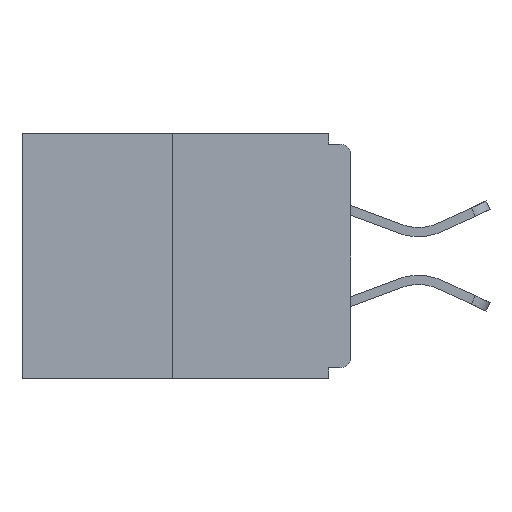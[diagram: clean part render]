
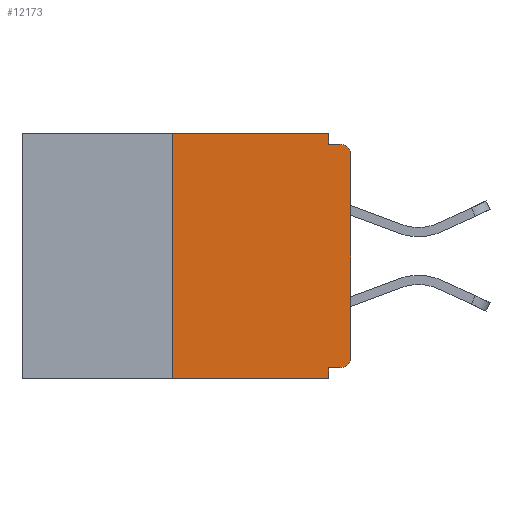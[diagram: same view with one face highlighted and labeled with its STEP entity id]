
A CAD part, left-side view. The second image highlights one B-rep face of the part: STEP entity #12173.
In plain terms, the highlighted planar face has unit normal (-1, 0, 0).
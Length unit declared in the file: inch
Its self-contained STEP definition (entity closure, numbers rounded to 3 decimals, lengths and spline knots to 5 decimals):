
#519 = VERTEX_POINT ( 'NONE', #11648 ) ;
#792 = VERTEX_POINT ( 'NONE', #8527 ) ;
#1219 = LINE ( 'NONE', #9843, #12576 ) ;
#1291 = CARTESIAN_POINT ( 'NONE',  ( 0., 0.25, 0. ) ) ;
#1317 = ORIENTED_EDGE ( 'NONE', *, *, #2907, .F. ) ;
#1701 = VERTEX_POINT ( 'NONE', #1969 ) ;
#1830 = CIRCLE ( 'NONE', #7094, 0.015 ) ;
#1933 = DIRECTION ( 'NONE',  ( -1., 0., 0. ) ) ;
#1969 = CARTESIAN_POINT ( 'NONE',  ( 0., 0.25, 0. ) ) ;
#2136 = ORIENTED_EDGE ( 'NONE', *, *, #7452, .T. ) ;
#2603 = CARTESIAN_POINT ( 'NONE',  ( 0., 0.25, -0.343 ) ) ;
#2713 = LINE ( 'NONE', #6133, #3054 ) ;
#2848 = FACE_OUTER_BOUND ( 'NONE', #6129, .T. ) ;
#2907 = EDGE_CURVE ( 'NONE', #4086, #519, #5922, .T. ) ;
#2918 = EDGE_CURVE ( 'NONE', #12275, #792, #8336, .T. ) ;
#2997 = DIRECTION ( 'NONE',  ( 0., 0., -1. ) ) ;
#3054 = VECTOR ( 'NONE', #9433, 39.37008 ) ;
#3148 = VECTOR ( 'NONE', #2997, 39.37008 ) ;
#3778 = CARTESIAN_POINT ( 'NONE',  ( 0., 0., -0.328 ) ) ;
#4086 = VERTEX_POINT ( 'NONE', #12281 ) ;
#4287 = CARTESIAN_POINT ( 'NONE',  ( 0., 0., -0.015 ) ) ;
#4357 = CARTESIAN_POINT ( 'NONE',  ( 0., 0.015, -0.03 ) ) ;
#4374 = DIRECTION ( 'NONE',  ( 0., -1., 0. ) ) ;
#4580 = CARTESIAN_POINT ( 'NONE',  ( 0., 0.015, -0.015 ) ) ;
#4688 = EDGE_CURVE ( 'NONE', #11669, #1701, #9485, .T. ) ;
#4873 = DIRECTION ( 'NONE',  ( 0., 1., 0. ) ) ;
#5019 = CARTESIAN_POINT ( 'NONE',  ( 0., 0.46, 0. ) ) ;
#5156 = CARTESIAN_POINT ( 'NONE',  ( 0., 0.031, -0.328 ) ) ;
#5581 = ORIENTED_EDGE ( 'NONE', *, *, #8995, .T. ) ;
#5749 = DIRECTION ( 'NONE',  ( 0., -1., 0. ) ) ;
#5922 = LINE ( 'NONE', #9660, #3148 ) ;
#6129 = EDGE_LOOP ( 'NONE', ( #10695, #13106, #13943, #7366, #12694, #10967, #5581, #2136, #9454, #1317 ) ) ;
#6133 = CARTESIAN_POINT ( 'NONE',  ( 0., 0.46, 0. ) ) ;
#6148 = DIRECTION ( 'NONE',  ( 0., 0., -1. ) ) ;
#6204 = PLANE ( 'NONE',  #9606 ) ;
#6557 = VECTOR ( 'NONE', #11391, 39.37008 ) ;
#6645 = EDGE_CURVE ( 'NONE', #1701, #4086, #2713, .T. ) ;
#6681 = VERTEX_POINT ( 'NONE', #7473 ) ;
#6757 = CARTESIAN_POINT ( 'NONE',  ( 0., 0.46, -0.343 ) ) ;
#7094 = AXIS2_PLACEMENT_3D ( 'NONE', #4357, #10989, #12197 ) ;
#7366 = ORIENTED_EDGE ( 'NONE', *, *, #8226, .F. ) ;
#7432 = VERTEX_POINT ( 'NONE', #7731 ) ;
#7452 = EDGE_CURVE ( 'NONE', #7432, #11315, #1830, .T. ) ;
#7473 = CARTESIAN_POINT ( 'NONE',  ( 0., 0.031, -0.343 ) ) ;
#7731 = CARTESIAN_POINT ( 'NONE',  ( 0., 0., -0.03 ) ) ;
#8181 = VERTEX_POINT ( 'NONE', #5156 ) ;
#8226 = EDGE_CURVE ( 'NONE', #8181, #6681, #1219, .T. ) ;
#8336 = CIRCLE ( 'NONE', #10806, 0.015 ) ;
#8390 = LINE ( 'NONE', #6757, #10610 ) ;
#8527 = CARTESIAN_POINT ( 'NONE',  ( 0., 0., -0.313 ) ) ;
#8888 = DIRECTION ( 'NONE',  ( 0., 0., -1. ) ) ;
#8995 = EDGE_CURVE ( 'NONE', #792, #7432, #13752, .T. ) ;
#9405 = DIRECTION ( 'NONE',  ( 1., 0., 0. ) ) ;
#9433 = DIRECTION ( 'NONE',  ( 0., -1., 0. ) ) ;
#9454 = ORIENTED_EDGE ( 'NONE', *, *, #9724, .F. ) ;
#9485 = LINE ( 'NONE', #1291, #6557 ) ;
#9606 = AXIS2_PLACEMENT_3D ( 'NONE', #5019, #9405, #6148 ) ;
#9660 = CARTESIAN_POINT ( 'NONE',  ( 0., 0.031, 0. ) ) ;
#9724 = EDGE_CURVE ( 'NONE', #519, #11315, #13924, .T. ) ;
#9841 = CARTESIAN_POINT ( 'NONE',  ( 0., 0.015, -0.328 ) ) ;
#9843 = CARTESIAN_POINT ( 'NONE',  ( 0., 0.031, -0.343 ) ) ;
#10417 = CARTESIAN_POINT ( 'NONE',  ( 0., 0., 0. ) ) ;
#10610 = VECTOR ( 'NONE', #5749, 39.37008 ) ;
#10695 = ORIENTED_EDGE ( 'NONE', *, *, #6645, .F. ) ;
#10726 = DIRECTION ( 'NONE',  ( 0., 0., -1. ) ) ;
#10773 = CARTESIAN_POINT ( 'NONE',  ( 0., 0.015, -0.313 ) ) ;
#10785 = EDGE_CURVE ( 'NONE', #12275, #8181, #13728, .T. ) ;
#10795 = VECTOR ( 'NONE', #4873, 39.37008 ) ;
#10806 = AXIS2_PLACEMENT_3D ( 'NONE', #10773, #1933, #10726 ) ;
#10967 = ORIENTED_EDGE ( 'NONE', *, *, #2918, .T. ) ;
#10989 = DIRECTION ( 'NONE',  ( -1., 0., 0. ) ) ;
#11002 = VECTOR ( 'NONE', #4374, 39.37008 ) ;
#11315 = VERTEX_POINT ( 'NONE', #4580 ) ;
#11318 = EDGE_CURVE ( 'NONE', #11669, #6681, #8390, .T. ) ;
#11391 = DIRECTION ( 'NONE',  ( 0., 0., 1. ) ) ;
#11648 = CARTESIAN_POINT ( 'NONE',  ( 0., 0.031, -0.015 ) ) ;
#11669 = VERTEX_POINT ( 'NONE', #2603 ) ;
#12173 = ADVANCED_FACE ( 'NONE', ( #2848 ), #6204, .F. ) ;
#12197 = DIRECTION ( 'NONE',  ( 0., 0., -1. ) ) ;
#12275 = VERTEX_POINT ( 'NONE', #9841 ) ;
#12281 = CARTESIAN_POINT ( 'NONE',  ( 0., 0.031, 0. ) ) ;
#12386 = VECTOR ( 'NONE', #12520, 39.37008 ) ;
#12520 = DIRECTION ( 'NONE',  ( 0., 0., 1. ) ) ;
#12576 = VECTOR ( 'NONE', #8888, 39.37008 ) ;
#12694 = ORIENTED_EDGE ( 'NONE', *, *, #10785, .F. ) ;
#13106 = ORIENTED_EDGE ( 'NONE', *, *, #4688, .F. ) ;
#13728 = LINE ( 'NONE', #3778, #10795 ) ;
#13752 = LINE ( 'NONE', #10417, #12386 ) ;
#13924 = LINE ( 'NONE', #4287, #11002 ) ;
#13943 = ORIENTED_EDGE ( 'NONE', *, *, #11318, .T. ) ;
